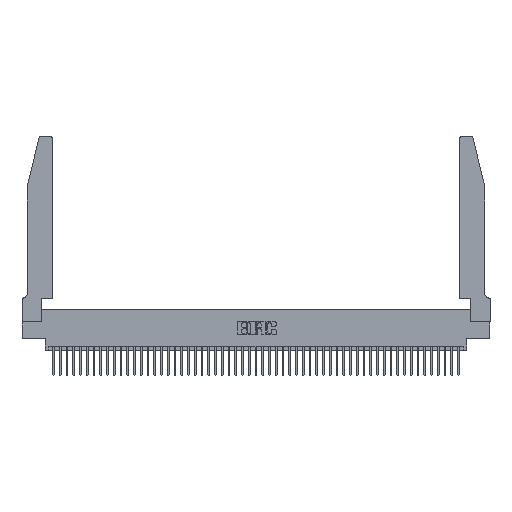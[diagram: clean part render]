
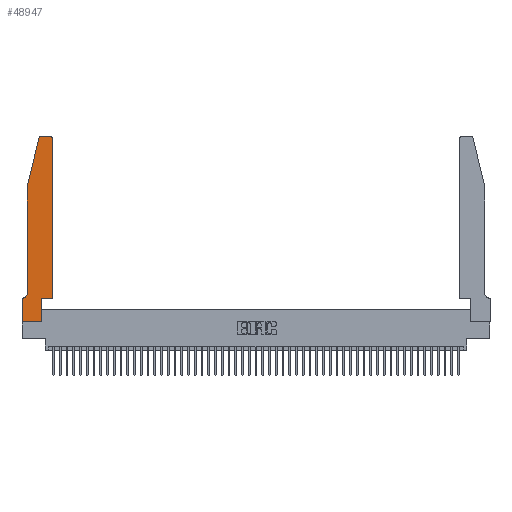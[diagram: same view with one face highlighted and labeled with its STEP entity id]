
A CAD part, top view. The second image highlights one B-rep face of the part: STEP entity #48947.
In plain terms, the highlighted planar face has unit normal (0, 0, 1).
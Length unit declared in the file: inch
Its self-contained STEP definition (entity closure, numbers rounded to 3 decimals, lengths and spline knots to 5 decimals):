
#101 = VERTEX_POINT ( 'NONE', #36163 ) ;
#285 = ORIENTED_EDGE ( 'NONE', *, *, #38076, .T. ) ;
#556 = VECTOR ( 'NONE', #49972, 39.37008 ) ;
#1355 = DIRECTION ( 'NONE',  ( -1., 0., 0. ) ) ;
#1815 = CARTESIAN_POINT ( 'NONE',  ( 0., 0., 0.37 ) ) ;
#2276 = EDGE_CURVE ( 'NONE', #22031, #36895, #22303, .T. ) ;
#2769 = CIRCLE ( 'NONE', #26478, 0.03 ) ;
#2874 = EDGE_CURVE ( 'NONE', #27434, #3854, #16155, .T. ) ;
#3845 = LINE ( 'NONE', #34198, #12970 ) ;
#3854 = VERTEX_POINT ( 'NONE', #30537 ) ;
#4780 = CARTESIAN_POINT ( 'NONE',  ( 0., 0., 0.37 ) ) ;
#4888 = EDGE_CURVE ( 'NONE', #36895, #5209, #40233, .T. ) ;
#5209 = VERTEX_POINT ( 'NONE', #10830 ) ;
#5277 = EDGE_CURVE ( 'NONE', #40908, #17728, #3845, .T. ) ;
#5370 = CARTESIAN_POINT ( 'NONE',  ( 0.0755, 0.35, 0.37 ) ) ;
#5652 = DIRECTION ( 'NONE',  ( 0., 0., 1. ) ) ;
#6199 = EDGE_CURVE ( 'NONE', #101, #27434, #43712, .T. ) ;
#6345 = LINE ( 'NONE', #28551, #45055 ) ;
#7258 = DIRECTION ( 'NONE',  ( 0., 1., 0. ) ) ;
#7373 = VERTEX_POINT ( 'NONE', #43427 ) ;
#7653 = VECTOR ( 'NONE', #32838, 39.37008 ) ;
#8082 = ORIENTED_EDGE ( 'NONE', *, *, #2276, .T. ) ;
#9359 = VECTOR ( 'NONE', #28758, 39.37008 ) ;
#9451 = PLANE ( 'NONE',  #27717 ) ;
#9684 = EDGE_LOOP ( 'NONE', ( #14717, #11703, #25673, #39528, #8082, #25723, #10570, #33018, #48738, #43310, #27081, #285 ) ) ;
#10570 = ORIENTED_EDGE ( 'NONE', *, *, #25672, .T. ) ;
#10830 = CARTESIAN_POINT ( 'NONE',  ( 0., 0.35, 0.37 ) ) ;
#11655 = DIRECTION ( 'NONE',  ( 0., 1., 0. ) ) ;
#11703 = ORIENTED_EDGE ( 'NONE', *, *, #6199, .T. ) ;
#11816 = VERTEX_POINT ( 'NONE', #44013 ) ;
#12599 = CARTESIAN_POINT ( 'NONE',  ( 0.4505, 0.35, 0.37 ) ) ;
#12970 = VECTOR ( 'NONE', #7258, 39.37008 ) ;
#13079 = VECTOR ( 'NONE', #11655, 39.37008 ) ;
#14227 = EDGE_CURVE ( 'NONE', #17728, #7373, #45894, .T. ) ;
#14717 = ORIENTED_EDGE ( 'NONE', *, *, #24946, .T. ) ;
#14947 = EDGE_CURVE ( 'NONE', #20744, #40908, #17964, .T. ) ;
#15881 = CARTESIAN_POINT ( 'NONE',  ( 0.4205, 2.72, 0.37 ) ) ;
#16155 = LINE ( 'NONE', #17579, #25272 ) ;
#16856 = FACE_OUTER_BOUND ( 'NONE', #9684, .T. ) ;
#17251 = DIRECTION ( 'NONE',  ( 1., 0., 0. ) ) ;
#17579 = CARTESIAN_POINT ( 'NONE',  ( 0.0755, 2., 0.37 ) ) ;
#17728 = VERTEX_POINT ( 'NONE', #43313 ) ;
#17964 = LINE ( 'NONE', #25098, #7653 ) ;
#18841 = EDGE_CURVE ( 'NONE', #3854, #22031, #40634, .T. ) ;
#19084 = CARTESIAN_POINT ( 'NONE',  ( 0.0755, 2., 0.37 ) ) ;
#19121 = CARTESIAN_POINT ( 'NONE',  ( 0.4505, 0.35, 0.37 ) ) ;
#19550 = CARTESIAN_POINT ( 'NONE',  ( 0.2865, 0., 0.37 ) ) ;
#19806 = DIRECTION ( 'NONE',  ( 1., 0., 0. ) ) ;
#20021 = CARTESIAN_POINT ( 'NONE',  ( 0.0055, 0.35, 0.37 ) ) ;
#20744 = VERTEX_POINT ( 'NONE', #4780 ) ;
#21064 = CARTESIAN_POINT ( 'NONE',  ( 0.0055, 0.42, 0.37 ) ) ;
#21460 = LINE ( 'NONE', #1815, #30496 ) ;
#22031 = VERTEX_POINT ( 'NONE', #39524 ) ;
#22303 = CIRCLE ( 'NONE', #39253, 0.07 ) ;
#22363 = VERTEX_POINT ( 'NONE', #34488 ) ;
#24946 = EDGE_CURVE ( 'NONE', #11816, #101, #6345, .T. ) ;
#24952 = DIRECTION ( 'NONE',  ( -1., 0., 0. ) ) ;
#25098 = CARTESIAN_POINT ( 'NONE',  ( 0., 0., 0.37 ) ) ;
#25272 = VECTOR ( 'NONE', #48494, 39.37008 ) ;
#25672 = EDGE_CURVE ( 'NONE', #5209, #20744, #21460, .T. ) ;
#25673 = ORIENTED_EDGE ( 'NONE', *, *, #2874, .T. ) ;
#25723 = ORIENTED_EDGE ( 'NONE', *, *, #4888, .T. ) ;
#26129 = AXIS2_PLACEMENT_3D ( 'NONE', #28867, #5652, #32758 ) ;
#26478 = AXIS2_PLACEMENT_3D ( 'NONE', #15881, #42916, #19806 ) ;
#26618 = VECTOR ( 'NONE', #35804, 39.37008 ) ;
#27081 = ORIENTED_EDGE ( 'NONE', *, *, #41971, .T. ) ;
#27434 = VERTEX_POINT ( 'NONE', #44706 ) ;
#27717 = AXIS2_PLACEMENT_3D ( 'NONE', #36548, #40407, #17251 ) ;
#28551 = CARTESIAN_POINT ( 'NONE',  ( 0.2605, 2.75, 0.37 ) ) ;
#28758 = DIRECTION ( 'NONE',  ( -1., 0., 0. ) ) ;
#28867 = CARTESIAN_POINT ( 'NONE',  ( 0.284, 2.72, 0.37 ) ) ;
#30496 = VECTOR ( 'NONE', #40636, 39.37008 ) ;
#30537 = CARTESIAN_POINT ( 'NONE',  ( 0.0755, 2., 0.37 ) ) ;
#32443 = LINE ( 'NONE', #19121, #13079 ) ;
#32758 = DIRECTION ( 'NONE',  ( 1., 0., 0. ) ) ;
#32838 = DIRECTION ( 'NONE',  ( 1., 0., 0. ) ) ;
#33018 = ORIENTED_EDGE ( 'NONE', *, *, #14947, .T. ) ;
#34198 = CARTESIAN_POINT ( 'NONE',  ( 0.2865, 0.35, 0.37 ) ) ;
#34488 = CARTESIAN_POINT ( 'NONE',  ( 0.4505, 2.72, 0.37 ) ) ;
#35804 = DIRECTION ( 'NONE',  ( 1., 0., 0. ) ) ;
#36163 = CARTESIAN_POINT ( 'NONE',  ( 0.284, 2.75, 0.37 ) ) ;
#36548 = CARTESIAN_POINT ( 'NONE',  ( 0., 0.35, 0.37 ) ) ;
#36895 = VERTEX_POINT ( 'NONE', #20021 ) ;
#38076 = EDGE_CURVE ( 'NONE', #22363, #11816, #2769, .T. ) ;
#39253 = AXIS2_PLACEMENT_3D ( 'NONE', #21064, #48043, #24952 ) ;
#39524 = CARTESIAN_POINT ( 'NONE',  ( 0.0755, 0.42, 0.37 ) ) ;
#39528 = ORIENTED_EDGE ( 'NONE', *, *, #18841, .T. ) ;
#40233 = LINE ( 'NONE', #5370, #9359 ) ;
#40407 = DIRECTION ( 'NONE',  ( 0., 0., 1. ) ) ;
#40634 = LINE ( 'NONE', #19084, #556 ) ;
#40636 = DIRECTION ( 'NONE',  ( 0., -1., 0. ) ) ;
#40908 = VERTEX_POINT ( 'NONE', #19550 ) ;
#41971 = EDGE_CURVE ( 'NONE', #7373, #22363, #32443, .T. ) ;
#42916 = DIRECTION ( 'NONE',  ( 0., 0., 1. ) ) ;
#43310 = ORIENTED_EDGE ( 'NONE', *, *, #14227, .T. ) ;
#43313 = CARTESIAN_POINT ( 'NONE',  ( 0.2865, 0.35, 0.37 ) ) ;
#43427 = CARTESIAN_POINT ( 'NONE',  ( 0.4505, 0.35, 0.37 ) ) ;
#43712 = CIRCLE ( 'NONE', #26129, 0.03 ) ;
#44013 = CARTESIAN_POINT ( 'NONE',  ( 0.4205, 2.75, 0.37 ) ) ;
#44706 = CARTESIAN_POINT ( 'NONE',  ( 0.25487, 2.72718, 0.37 ) ) ;
#45055 = VECTOR ( 'NONE', #1355, 39.37008 ) ;
#45894 = LINE ( 'NONE', #12599, #26618 ) ;
#48043 = DIRECTION ( 'NONE',  ( 0., 0., -1. ) ) ;
#48494 = DIRECTION ( 'NONE',  ( -0.239, -0.971, 0. ) ) ;
#48738 = ORIENTED_EDGE ( 'NONE', *, *, #5277, .T. ) ;
#48947 = ADVANCED_FACE ( 'NONE', ( #16856 ), #9451, .T. ) ;
#49972 = DIRECTION ( 'NONE',  ( 0., -1., 0. ) ) ;
